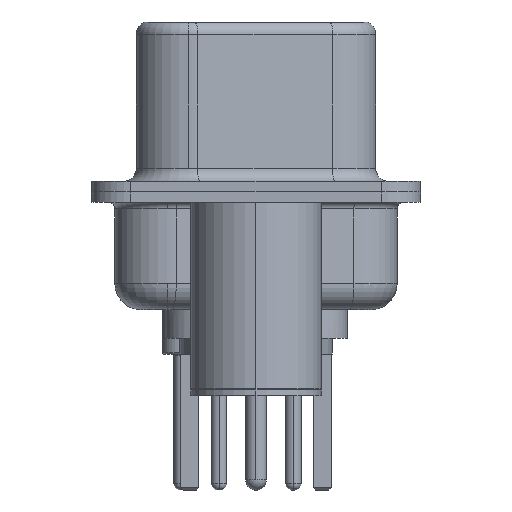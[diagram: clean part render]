
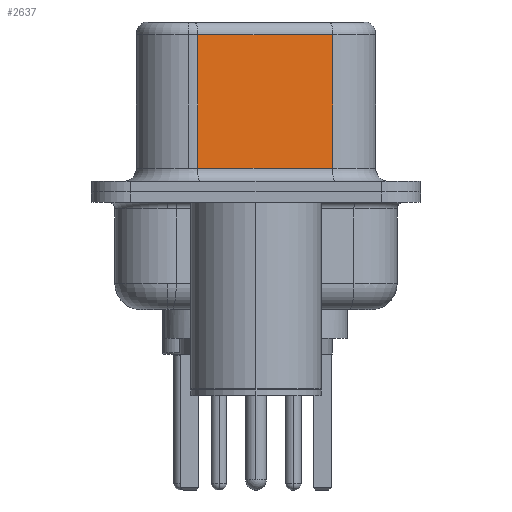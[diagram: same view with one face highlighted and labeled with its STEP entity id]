
A CAD part, left-side view. The second image highlights one B-rep face of the part: STEP entity #2637.
In plain terms, the highlighted planar face has unit normal (-0.985, -0.174, 0).
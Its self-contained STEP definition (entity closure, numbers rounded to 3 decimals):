
#1009 = DIRECTION ( 'NONE',  ( 0., 0., -1. ) ) ;
#1501 = VERTEX_POINT ( 'NONE', #3210 ) ;
#1958 = DIRECTION ( 'NONE',  ( 0., 0., -1. ) ) ;
#2074 = VECTOR ( 'NONE', #6298, 1000. ) ;
#2637 = ADVANCED_FACE ( 'NONE', ( #7608 ), #26273, .F. ) ;
#3210 = CARTESIAN_POINT ( 'NONE',  ( 3.675, 2.233, 0.9 ) ) ;
#3476 = VECTOR ( 'NONE', #17646, 1000. ) ;
#3931 = VERTEX_POINT ( 'NONE', #9756 ) ;
#4111 = AXIS2_PLACEMENT_3D ( 'NONE', #24318, #5005, #15716 ) ;
#5005 = DIRECTION ( 'NONE',  ( 0.985, 0.174, 0. ) ) ;
#5417 = LINE ( 'NONE', #23392, #2074 ) ;
#6298 = DIRECTION ( 'NONE',  ( -0.174, 0.985, 0. ) ) ;
#7608 = FACE_OUTER_BOUND ( 'NONE', #25346, .T. ) ;
#9123 = LINE ( 'NONE', #15804, #3476 ) ;
#9710 = ORIENTED_EDGE ( 'NONE', *, *, #15434, .T. ) ;
#9756 = CARTESIAN_POINT ( 'NONE',  ( 3.675, 2.233, 6.02 ) ) ;
#11707 = LINE ( 'NONE', #18601, #26281 ) ;
#12620 = EDGE_CURVE ( 'NONE', #25836, #15203, #27004, .T. ) ;
#13100 = CARTESIAN_POINT ( 'NONE',  ( 4.585, -2.927, 6.02 ) ) ;
#13427 = CARTESIAN_POINT ( 'NONE',  ( 4.585, -2.927, 6.52 ) ) ;
#14171 = ORIENTED_EDGE ( 'NONE', *, *, #15602, .T. ) ;
#15203 = VERTEX_POINT ( 'NONE', #20155 ) ;
#15434 = EDGE_CURVE ( 'NONE', #3931, #1501, #11707, .T. ) ;
#15602 = EDGE_CURVE ( 'NONE', #25836, #3931, #5417, .T. ) ;
#15716 = DIRECTION ( 'NONE',  ( -0.174, 0.985, 0. ) ) ;
#15804 = CARTESIAN_POINT ( 'NONE',  ( 4.585, -2.927, 0.9 ) ) ;
#17646 = DIRECTION ( 'NONE',  ( 0.174, -0.985, 0. ) ) ;
#18601 = CARTESIAN_POINT ( 'NONE',  ( 3.675, 2.233, 6.52 ) ) ;
#20155 = CARTESIAN_POINT ( 'NONE',  ( 4.585, -2.927, 0.9 ) ) ;
#22271 = EDGE_CURVE ( 'NONE', #1501, #15203, #9123, .T. ) ;
#23392 = CARTESIAN_POINT ( 'NONE',  ( 4.585, -2.927, 6.02 ) ) ;
#24120 = ORIENTED_EDGE ( 'NONE', *, *, #12620, .F. ) ;
#24318 = CARTESIAN_POINT ( 'NONE',  ( 4.585, -2.927, 6.52 ) ) ;
#25004 = VECTOR ( 'NONE', #1009, 1000. ) ;
#25346 = EDGE_LOOP ( 'NONE', ( #24120, #14171, #9710, #26528 ) ) ;
#25836 = VERTEX_POINT ( 'NONE', #13100 ) ;
#26273 = PLANE ( 'NONE',  #4111 ) ;
#26281 = VECTOR ( 'NONE', #1958, 1000. ) ;
#26528 = ORIENTED_EDGE ( 'NONE', *, *, #22271, .T. ) ;
#27004 = LINE ( 'NONE', #13427, #25004 ) ;
